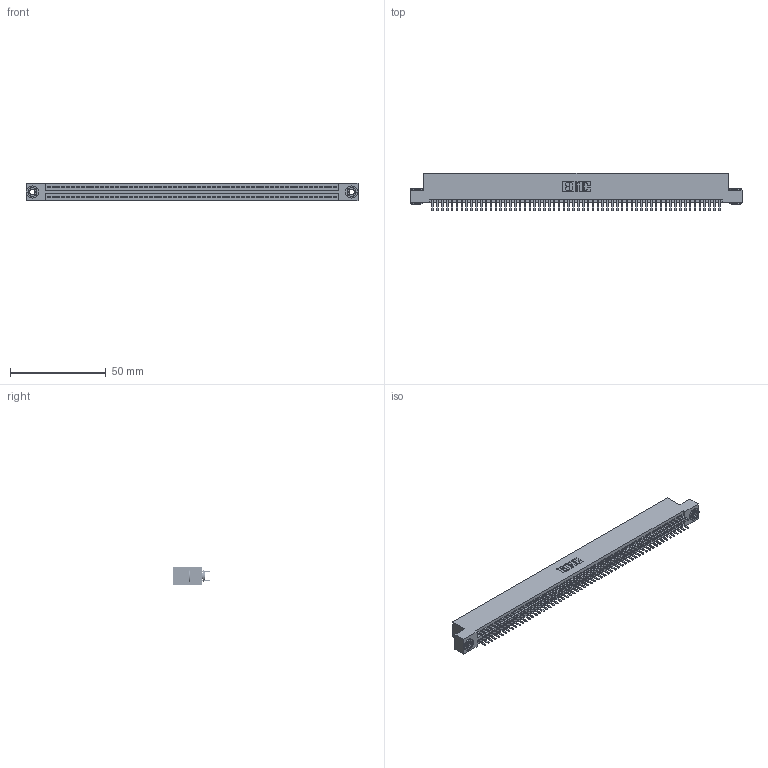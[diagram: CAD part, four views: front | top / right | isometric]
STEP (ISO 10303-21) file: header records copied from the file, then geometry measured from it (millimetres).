
FILE_DESCRIPTION (( 'STEP AP203' ), '1' );
FILE_NAME ('845-120-520-203.STEP', '2018-11-21T01:00:50', ( '' ), ( '' ), 'SwSTEP 2.0', 'SolidWorks 2016', '' );
FILE_SCHEMA (( 'CONFIG_CONTROL_DESIGN' ));
Length unit declared in the file: inch
Products named in the file (4): 845 Part_Flush Mounting Lugs - 0.156 Dia-TH; 345-292-001_345-293-120; 345-250-002_345-250-002-102; 845-120-520-203
Assembly tree (123 placements, depth 2):
  845-120-520-203
    845 Part_Flush Mounting Lugs - 0.156 Dia-TH
    345-292-001_345-293-120  x120
    345-250-002_345-250-002-102  x2
Bounding box: 173.61 x 19.68 x 9.4 mm (x, y, z)
Volume: 16998.3 mm3; surface area: 25567.6 mm2
Topology: 123 solids, 123 shells, 6644 faces, 19257 edges, 12514 vertices
Faces by surface type: plane 4290, cylinder 2346, cone 8
Entity records: 45418 total; most frequent: CARTESIAN_POINT 7583, ORIENTED_EDGE 7498, DIRECTION 6683, EDGE_CURVE 3749, LINE 3349, VECTOR 3349, VERTEX_POINT 2494, AXIS2_PLACEMENT_3D 1667
